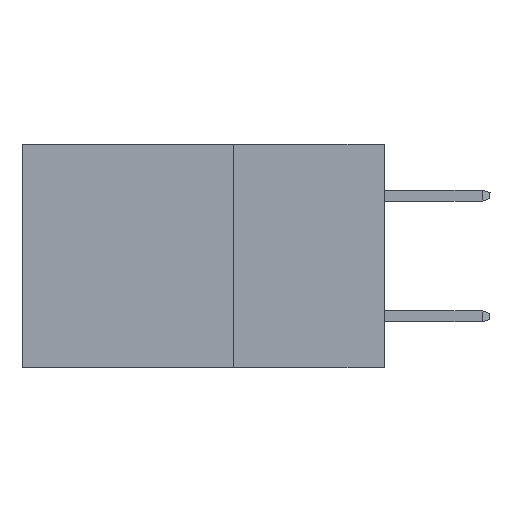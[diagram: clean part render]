
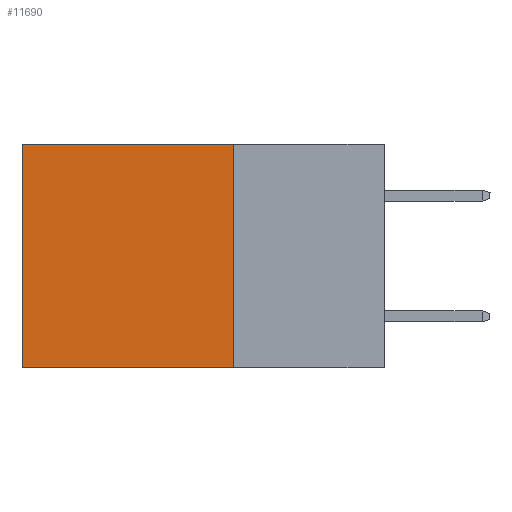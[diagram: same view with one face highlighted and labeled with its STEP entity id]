
A CAD part, left-side view. The second image highlights one B-rep face of the part: STEP entity #11690.
In plain terms, the highlighted planar face has unit normal (-1, 0, 0).
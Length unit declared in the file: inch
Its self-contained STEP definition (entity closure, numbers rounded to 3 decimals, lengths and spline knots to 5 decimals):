
#339 = LINE ( 'NONE', #5069, #16557 ) ;
#996 = ORIENTED_EDGE ( 'NONE', *, *, #2612, .F. ) ;
#1726 = DIRECTION ( 'NONE',  ( 0., 1., 0. ) ) ;
#2542 = CARTESIAN_POINT ( 'NONE',  ( 0.298, 0.6, -0.37 ) ) ;
#2577 = VERTEX_POINT ( 'NONE', #7310 ) ;
#2612 = EDGE_CURVE ( 'NONE', #2577, #3069, #16013, .T. ) ;
#2918 = PLANE ( 'NONE',  #7622 ) ;
#2938 = ORIENTED_EDGE ( 'NONE', *, *, #5123, .T. ) ;
#3069 = VERTEX_POINT ( 'NONE', #18372 ) ;
#3391 = LINE ( 'NONE', #7599, #11234 ) ;
#4336 = CARTESIAN_POINT ( 'NONE',  ( 0.298, 0.25, 0. ) ) ;
#4715 = ORIENTED_EDGE ( 'NONE', *, *, #13701, .T. ) ;
#5069 = CARTESIAN_POINT ( 'NONE',  ( 0.298, 0.6, 0. ) ) ;
#5123 = EDGE_CURVE ( 'NONE', #2577, #8454, #3391, .T. ) ;
#5134 = DIRECTION ( 'NONE',  ( 0., 0., -1. ) ) ;
#6037 = CARTESIAN_POINT ( 'NONE',  ( 0.298, 0.6, 0. ) ) ;
#6578 = LINE ( 'NONE', #9384, #16403 ) ;
#7310 = CARTESIAN_POINT ( 'NONE',  ( 0.298, 0.25, 0. ) ) ;
#7382 = DIRECTION ( 'NONE',  ( 0., 0., -1. ) ) ;
#7593 = VERTEX_POINT ( 'NONE', #2542 ) ;
#7599 = CARTESIAN_POINT ( 'NONE',  ( 0.298, 0.25, 0. ) ) ;
#7622 = AXIS2_PLACEMENT_3D ( 'NONE', #13917, #18580, #10663 ) ;
#8454 = VERTEX_POINT ( 'NONE', #6037 ) ;
#9248 = DIRECTION ( 'NONE',  ( 0., 1., 0. ) ) ;
#9384 = CARTESIAN_POINT ( 'NONE',  ( 0.298, 0.25, -0.37 ) ) ;
#10663 = DIRECTION ( 'NONE',  ( 0., 0., -1. ) ) ;
#10880 = EDGE_LOOP ( 'NONE', ( #4715, #17764, #996, #2938 ) ) ;
#11234 = VECTOR ( 'NONE', #9248, 39.37008 ) ;
#11283 = EDGE_CURVE ( 'NONE', #3069, #7593, #6578, .T. ) ;
#11486 = FACE_OUTER_BOUND ( 'NONE', #10880, .T. ) ;
#11690 = ADVANCED_FACE ( 'NONE', ( #11486 ), #2918, .F. ) ;
#13701 = EDGE_CURVE ( 'NONE', #8454, #7593, #339, .T. ) ;
#13917 = CARTESIAN_POINT ( 'NONE',  ( 0.298, 0.25, 0. ) ) ;
#16013 = LINE ( 'NONE', #4336, #19201 ) ;
#16403 = VECTOR ( 'NONE', #1726, 39.37008 ) ;
#16557 = VECTOR ( 'NONE', #5134, 39.37008 ) ;
#17764 = ORIENTED_EDGE ( 'NONE', *, *, #11283, .F. ) ;
#18372 = CARTESIAN_POINT ( 'NONE',  ( 0.298, 0.25, -0.37 ) ) ;
#18580 = DIRECTION ( 'NONE',  ( 1., 0., 0. ) ) ;
#19201 = VECTOR ( 'NONE', #7382, 39.37008 ) ;
